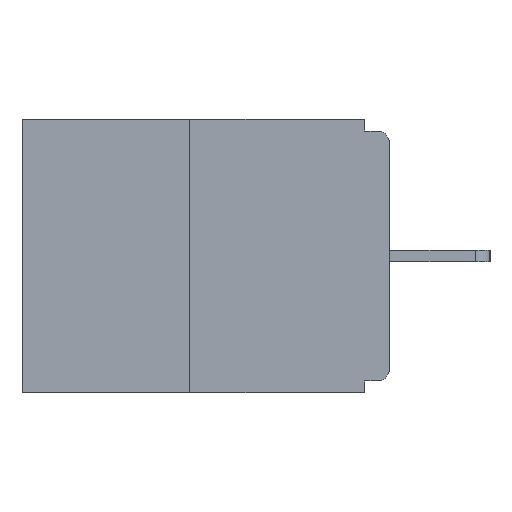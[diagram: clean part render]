
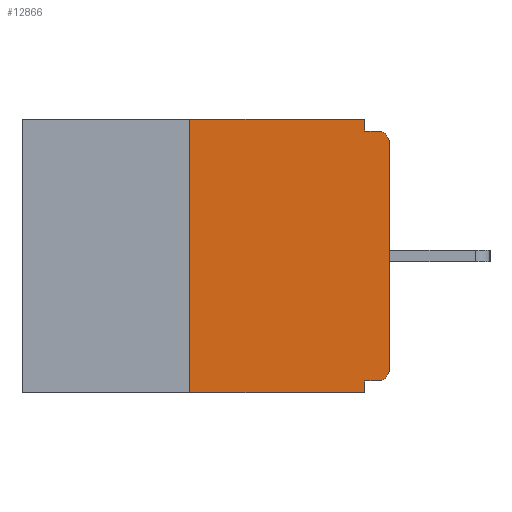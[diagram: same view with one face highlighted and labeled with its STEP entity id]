
A CAD part, left-side view. The second image highlights one B-rep face of the part: STEP entity #12866.
In plain terms, the highlighted planar face has unit normal (-1, 0, 0).
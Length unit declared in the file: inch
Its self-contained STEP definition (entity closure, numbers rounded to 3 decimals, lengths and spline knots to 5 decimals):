
#188 = CARTESIAN_POINT ( 'NONE',  ( 0., 0.015, -0.313 ) ) ;
#222 = LINE ( 'NONE', #17030, #15788 ) ;
#830 = DIRECTION ( 'NONE',  ( 0., 0., -1. ) ) ;
#971 = ORIENTED_EDGE ( 'NONE', *, *, #13811, .F. ) ;
#1449 = CARTESIAN_POINT ( 'NONE',  ( 0., 0.031, -0.015 ) ) ;
#1602 = AXIS2_PLACEMENT_3D ( 'NONE', #188, #5369, #6921 ) ;
#1965 = VECTOR ( 'NONE', #2068, 39.37008 ) ;
#2068 = DIRECTION ( 'NONE',  ( 0., 1., 0. ) ) ;
#2524 = VERTEX_POINT ( 'NONE', #13057 ) ;
#2533 = VERTEX_POINT ( 'NONE', #1449 ) ;
#2942 = CARTESIAN_POINT ( 'NONE',  ( 0., 0.46, 0. ) ) ;
#2978 = CARTESIAN_POINT ( 'NONE',  ( 0., 0.25, 0. ) ) ;
#3069 = EDGE_CURVE ( 'NONE', #14540, #17192, #15341, .T. ) ;
#3088 = EDGE_CURVE ( 'NONE', #14540, #8180, #19252, .T. ) ;
#3481 = ORIENTED_EDGE ( 'NONE', *, *, #11473, .F. ) ;
#4277 = CARTESIAN_POINT ( 'NONE',  ( 0., 0., -0.03 ) ) ;
#4491 = CARTESIAN_POINT ( 'NONE',  ( 0., 0.031, -0.328 ) ) ;
#5019 = ORIENTED_EDGE ( 'NONE', *, *, #19658, .F. ) ;
#5254 = DIRECTION ( 'NONE',  ( 0., 0., -1. ) ) ;
#5369 = DIRECTION ( 'NONE',  ( -1., 0., 0. ) ) ;
#5883 = ORIENTED_EDGE ( 'NONE', *, *, #3069, .F. ) ;
#6213 = AXIS2_PLACEMENT_3D ( 'NONE', #13062, #15152, #21890 ) ;
#6464 = EDGE_CURVE ( 'NONE', #19491, #20958, #6556, .T. ) ;
#6556 = CIRCLE ( 'NONE', #6213, 0.015 ) ;
#6783 = ORIENTED_EDGE ( 'NONE', *, *, #7715, .F. ) ;
#6824 = ORIENTED_EDGE ( 'NONE', *, *, #17051, .T. ) ;
#6847 = VECTOR ( 'NONE', #11455, 39.37008 ) ;
#6907 = LINE ( 'NONE', #20423, #18023 ) ;
#6921 = DIRECTION ( 'NONE',  ( 0., 0., -1. ) ) ;
#7553 = CARTESIAN_POINT ( 'NONE',  ( 0., 0.46, -0.343 ) ) ;
#7715 = EDGE_CURVE ( 'NONE', #20853, #10787, #222, .T. ) ;
#7961 = CARTESIAN_POINT ( 'NONE',  ( 0., 0., 0. ) ) ;
#8041 = LINE ( 'NONE', #21570, #18038 ) ;
#8180 = VERTEX_POINT ( 'NONE', #14008 ) ;
#8674 = EDGE_CURVE ( 'NONE', #8180, #19491, #9299, .T. ) ;
#9299 = LINE ( 'NONE', #7961, #15766 ) ;
#9307 = VECTOR ( 'NONE', #9898, 39.37008 ) ;
#9458 = ORIENTED_EDGE ( 'NONE', *, *, #20904, .F. ) ;
#9665 = VECTOR ( 'NONE', #14089, 39.37008 ) ;
#9898 = DIRECTION ( 'NONE',  ( 0., -1., 0. ) ) ;
#10563 = CARTESIAN_POINT ( 'NONE',  ( 0., 0.46, 0. ) ) ;
#10784 = PLANE ( 'NONE',  #11650 ) ;
#10787 = VERTEX_POINT ( 'NONE', #2978 ) ;
#11237 = LINE ( 'NONE', #2942, #6847 ) ;
#11455 = DIRECTION ( 'NONE',  ( 0., -1., 0. ) ) ;
#11473 = EDGE_CURVE ( 'NONE', #19548, #2533, #6907, .T. ) ;
#11650 = AXIS2_PLACEMENT_3D ( 'NONE', #10563, #19182, #830 ) ;
#12543 = LINE ( 'NONE', #7553, #9665 ) ;
#12729 = DIRECTION ( 'NONE',  ( 0., 0., 1. ) ) ;
#12796 = ORIENTED_EDGE ( 'NONE', *, *, #3088, .T. ) ;
#12866 = ADVANCED_FACE ( 'NONE', ( #20536 ), #10784, .F. ) ;
#13057 = CARTESIAN_POINT ( 'NONE',  ( 0., 0.031, -0.343 ) ) ;
#13062 = CARTESIAN_POINT ( 'NONE',  ( 0., 0.015, -0.03 ) ) ;
#13811 = EDGE_CURVE ( 'NONE', #17192, #2524, #8041, .T. ) ;
#14008 = CARTESIAN_POINT ( 'NONE',  ( 0., 0., -0.313 ) ) ;
#14089 = DIRECTION ( 'NONE',  ( 0., -1., 0. ) ) ;
#14540 = VERTEX_POINT ( 'NONE', #20635 ) ;
#15152 = DIRECTION ( 'NONE',  ( -1., 0., 0. ) ) ;
#15341 = LINE ( 'NONE', #17216, #1965 ) ;
#15373 = DIRECTION ( 'NONE',  ( 0., 0., 1. ) ) ;
#15766 = VECTOR ( 'NONE', #12729, 39.37008 ) ;
#15788 = VECTOR ( 'NONE', #15373, 39.37008 ) ;
#16656 = LINE ( 'NONE', #18309, #9307 ) ;
#17030 = CARTESIAN_POINT ( 'NONE',  ( 0., 0.25, 0. ) ) ;
#17051 = EDGE_CURVE ( 'NONE', #20853, #2524, #12543, .T. ) ;
#17192 = VERTEX_POINT ( 'NONE', #4491 ) ;
#17216 = CARTESIAN_POINT ( 'NONE',  ( 0., 0., -0.328 ) ) ;
#17738 = ORIENTED_EDGE ( 'NONE', *, *, #8674, .T. ) ;
#17991 = CARTESIAN_POINT ( 'NONE',  ( 0., 0.25, -0.343 ) ) ;
#18023 = VECTOR ( 'NONE', #5254, 39.37008 ) ;
#18038 = VECTOR ( 'NONE', #19899, 39.37008 ) ;
#18062 = ORIENTED_EDGE ( 'NONE', *, *, #6464, .T. ) ;
#18309 = CARTESIAN_POINT ( 'NONE',  ( 0., 0., -0.015 ) ) ;
#18414 = CARTESIAN_POINT ( 'NONE',  ( 0., 0.031, 0. ) ) ;
#19182 = DIRECTION ( 'NONE',  ( 1., 0., 0. ) ) ;
#19252 = CIRCLE ( 'NONE', #1602, 0.015 ) ;
#19491 = VERTEX_POINT ( 'NONE', #4277 ) ;
#19548 = VERTEX_POINT ( 'NONE', #18414 ) ;
#19658 = EDGE_CURVE ( 'NONE', #2533, #20958, #16656, .T. ) ;
#19899 = DIRECTION ( 'NONE',  ( 0., 0., -1. ) ) ;
#20088 = CARTESIAN_POINT ( 'NONE',  ( 0., 0.015, -0.015 ) ) ;
#20285 = EDGE_LOOP ( 'NONE', ( #9458, #6783, #6824, #971, #5883, #12796, #17738, #18062, #5019, #3481 ) ) ;
#20423 = CARTESIAN_POINT ( 'NONE',  ( 0., 0.031, 0. ) ) ;
#20536 = FACE_OUTER_BOUND ( 'NONE', #20285, .T. ) ;
#20635 = CARTESIAN_POINT ( 'NONE',  ( 0., 0.015, -0.328 ) ) ;
#20853 = VERTEX_POINT ( 'NONE', #17991 ) ;
#20904 = EDGE_CURVE ( 'NONE', #10787, #19548, #11237, .T. ) ;
#20958 = VERTEX_POINT ( 'NONE', #20088 ) ;
#21570 = CARTESIAN_POINT ( 'NONE',  ( 0., 0.031, -0.343 ) ) ;
#21890 = DIRECTION ( 'NONE',  ( 0., 0., -1. ) ) ;
